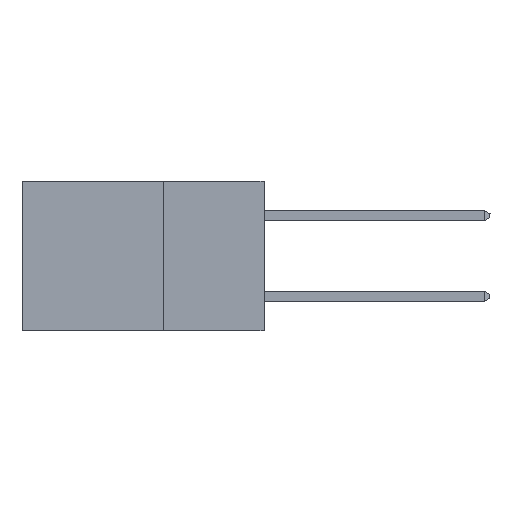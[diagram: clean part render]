
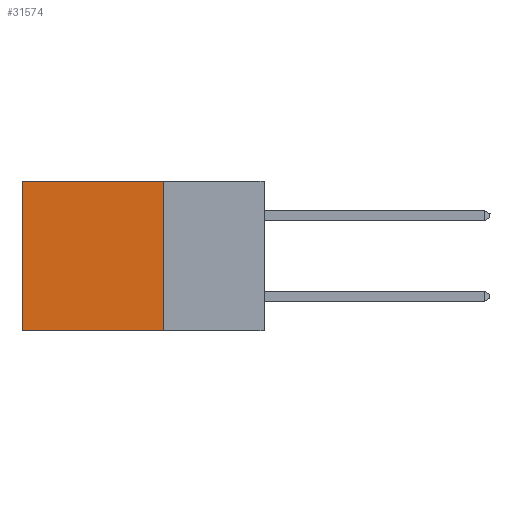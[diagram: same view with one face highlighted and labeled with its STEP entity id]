
A CAD part, left-side view. The second image highlights one B-rep face of the part: STEP entity #31574.
In plain terms, the highlighted planar face has unit normal (-1, 0, 0).
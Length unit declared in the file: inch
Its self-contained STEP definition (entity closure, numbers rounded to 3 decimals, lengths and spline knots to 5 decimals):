
#49 = VERTEX_POINT ( 'NONE', #537 ) ;
#109 = VERTEX_POINT ( 'NONE', #32370 ) ;
#537 = CARTESIAN_POINT ( 'NONE',  ( 0.298, 0.25, 0. ) ) ;
#844 = ORIENTED_EDGE ( 'NONE', *, *, #9917, .T. ) ;
#1361 = ORIENTED_EDGE ( 'NONE', *, *, #30061, .F. ) ;
#1587 = VERTEX_POINT ( 'NONE', #19335 ) ;
#1637 = CARTESIAN_POINT ( 'NONE',  ( 0.298, 0.6, 0. ) ) ;
#1985 = VECTOR ( 'NONE', #28781, 39.37008 ) ;
#3197 = CARTESIAN_POINT ( 'NONE',  ( 0.298, 0.25, 0. ) ) ;
#4915 = CARTESIAN_POINT ( 'NONE',  ( 0.298, 0.25, 0. ) ) ;
#7197 = VERTEX_POINT ( 'NONE', #14440 ) ;
#7749 = VECTOR ( 'NONE', #17562, 39.37008 ) ;
#9917 = EDGE_CURVE ( 'NONE', #49, #109, #30135, .T. ) ;
#12775 = VECTOR ( 'NONE', #29734, 39.37008 ) ;
#13457 = PLANE ( 'NONE',  #20417 ) ;
#13567 = DIRECTION ( 'NONE',  ( 0., 0., -1. ) ) ;
#14379 = FACE_OUTER_BOUND ( 'NONE', #30293, .T. ) ;
#14440 = CARTESIAN_POINT ( 'NONE',  ( 0.298, 0.25, -0.37 ) ) ;
#16959 = ORIENTED_EDGE ( 'NONE', *, *, #24167, .T. ) ;
#17562 = DIRECTION ( 'NONE',  ( 0., 1., 0. ) ) ;
#17584 = VECTOR ( 'NONE', #29437, 39.37008 ) ;
#19335 = CARTESIAN_POINT ( 'NONE',  ( 0.298, 0.6, -0.37 ) ) ;
#19454 = LINE ( 'NONE', #27257, #12775 ) ;
#20417 = AXIS2_PLACEMENT_3D ( 'NONE', #3197, #28545, #13567 ) ;
#22967 = LINE ( 'NONE', #23745, #1985 ) ;
#23745 = CARTESIAN_POINT ( 'NONE',  ( 0.298, 0.25, -0.37 ) ) ;
#24167 = EDGE_CURVE ( 'NONE', #109, #1587, #24186, .T. ) ;
#24186 = LINE ( 'NONE', #1637, #17584 ) ;
#27257 = CARTESIAN_POINT ( 'NONE',  ( 0.298, 0.25, 0. ) ) ;
#28545 = DIRECTION ( 'NONE',  ( 1., 0., 0. ) ) ;
#28638 = ORIENTED_EDGE ( 'NONE', *, *, #30336, .F. ) ;
#28781 = DIRECTION ( 'NONE',  ( 0., 1., 0. ) ) ;
#29437 = DIRECTION ( 'NONE',  ( 0., 0., -1. ) ) ;
#29734 = DIRECTION ( 'NONE',  ( 0., 0., -1. ) ) ;
#30061 = EDGE_CURVE ( 'NONE', #7197, #1587, #22967, .T. ) ;
#30135 = LINE ( 'NONE', #4915, #7749 ) ;
#30293 = EDGE_LOOP ( 'NONE', ( #16959, #1361, #28638, #844 ) ) ;
#30336 = EDGE_CURVE ( 'NONE', #49, #7197, #19454, .T. ) ;
#31574 = ADVANCED_FACE ( 'NONE', ( #14379 ), #13457, .F. ) ;
#32370 = CARTESIAN_POINT ( 'NONE',  ( 0.298, 0.6, 0. ) ) ;
